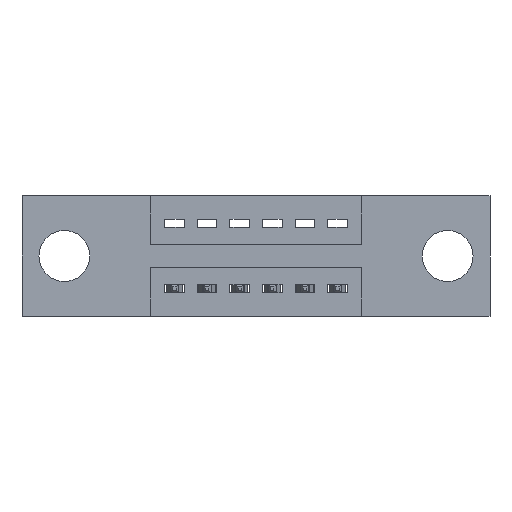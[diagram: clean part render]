
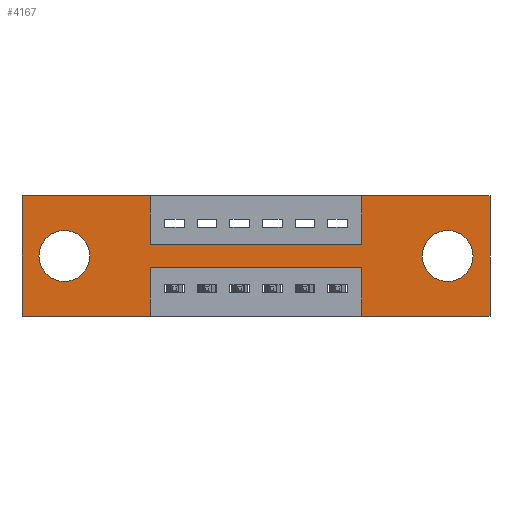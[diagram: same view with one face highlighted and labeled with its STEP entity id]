
A CAD part, front view. The second image highlights one B-rep face of the part: STEP entity #4167.
In plain terms, the highlighted planar face has unit normal (0, -1, 0).
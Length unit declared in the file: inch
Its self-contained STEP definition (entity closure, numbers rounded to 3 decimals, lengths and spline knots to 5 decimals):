
#25 = DIRECTION ( 'NONE',  ( 0., 0., -1. ) ) ;
#95 = EDGE_CURVE ( 'NONE', #3521, #7175, #1944, .T. ) ;
#239 = CIRCLE ( 'NONE', #1973, 0.078 ) ;
#276 = EDGE_CURVE ( 'NONE', #5040, #4251, #2736, .T. ) ;
#314 = LINE ( 'NONE', #8719, #5514 ) ;
#422 = CARTESIAN_POINT ( 'NONE',  ( 0.3925, 0., -0.15 ) ) ;
#449 = EDGE_CURVE ( 'NONE', #4128, #1882, #5234, .T. ) ;
#519 = VECTOR ( 'NONE', #3406, 39.37008 ) ;
#688 = VERTEX_POINT ( 'NONE', #8047 ) ;
#739 = EDGE_CURVE ( 'NONE', #4706, #4128, #9322, .T. ) ;
#760 = CARTESIAN_POINT ( 'NONE',  ( 0.13, 0., -0.107 ) ) ;
#782 = AXIS2_PLACEMENT_3D ( 'NONE', #5456, #6275, #2600 ) ;
#1037 = DIRECTION ( 'NONE',  ( 0., 1., 0. ) ) ;
#1062 = VECTOR ( 'NONE', #7769, 39.37008 ) ;
#1063 = DIRECTION ( 'NONE',  ( 0., 0., 1. ) ) ;
#1074 = CARTESIAN_POINT ( 'NONE',  ( 0.3925, 0., -0.15 ) ) ;
#1185 = VECTOR ( 'NONE', #4696, 39.37008 ) ;
#1388 = EDGE_CURVE ( 'NONE', #6924, #5683, #239, .T. ) ;
#1399 = CARTESIAN_POINT ( 'NONE',  ( 1.435, 0., 0. ) ) ;
#1438 = ORIENTED_EDGE ( 'NONE', *, *, #8268, .F. ) ;
#1604 = DIRECTION ( 'NONE',  ( -1., 0., 0. ) ) ;
#1612 = PLANE ( 'NONE',  #6044 ) ;
#1666 = CIRCLE ( 'NONE', #8547, 0.078 ) ;
#1681 = DIRECTION ( 'NONE',  ( 1., 0., 0. ) ) ;
#1755 = DIRECTION ( 'NONE',  ( 0., 0., -1. ) ) ;
#1757 = ORIENTED_EDGE ( 'NONE', *, *, #1388, .T. ) ;
#1793 = CARTESIAN_POINT ( 'NONE',  ( 1.0425, 0., 0. ) ) ;
#1882 = VERTEX_POINT ( 'NONE', #5999 ) ;
#1934 = VECTOR ( 'NONE', #6250, 39.37008 ) ;
#1942 = CARTESIAN_POINT ( 'NONE',  ( 1.0425, 0., -0.37 ) ) ;
#1944 = LINE ( 'NONE', #9113, #5788 ) ;
#1973 = AXIS2_PLACEMENT_3D ( 'NONE', #6489, #5694, #5533 ) ;
#1988 = ORIENTED_EDGE ( 'NONE', *, *, #3425, .T. ) ;
#2092 = EDGE_LOOP ( 'NONE', ( #8582, #7109 ) ) ;
#2097 = VERTEX_POINT ( 'NONE', #422 ) ;
#2261 = VERTEX_POINT ( 'NONE', #7986 ) ;
#2283 = CARTESIAN_POINT ( 'NONE',  ( 0.13, 0., -0.263 ) ) ;
#2379 = EDGE_CURVE ( 'NONE', #688, #2999, #2798, .T. ) ;
#2382 = CARTESIAN_POINT ( 'NONE',  ( 0., 0., -0.37 ) ) ;
#2531 = ORIENTED_EDGE ( 'NONE', *, *, #739, .F. ) ;
#2545 = DIRECTION ( 'NONE',  ( -1., 0., 0. ) ) ;
#2600 = DIRECTION ( 'NONE',  ( 0., 0., -1. ) ) ;
#2736 = LINE ( 'NONE', #6894, #4638 ) ;
#2756 = LINE ( 'NONE', #4491, #7088 ) ;
#2798 = CIRCLE ( 'NONE', #782, 0.078 ) ;
#2875 = FACE_BOUND ( 'NONE', #3535, .T. ) ;
#2947 = CARTESIAN_POINT ( 'NONE',  ( 0., 0., -0.37 ) ) ;
#2999 = VERTEX_POINT ( 'NONE', #8835 ) ;
#3116 = DIRECTION ( 'NONE',  ( 0., 0., -1. ) ) ;
#3144 = EDGE_CURVE ( 'NONE', #8443, #4706, #314, .T. ) ;
#3175 = DIRECTION ( 'NONE',  ( 0., -1., 0. ) ) ;
#3232 = CARTESIAN_POINT ( 'NONE',  ( 1.0425, 0., -0.15 ) ) ;
#3284 = ORIENTED_EDGE ( 'NONE', *, *, #5875, .F. ) ;
#3406 = DIRECTION ( 'NONE',  ( -1., 0., 0. ) ) ;
#3425 = EDGE_CURVE ( 'NONE', #5683, #6924, #1666, .T. ) ;
#3469 = CARTESIAN_POINT ( 'NONE',  ( 0.3925, 0., -0.37 ) ) ;
#3513 = EDGE_CURVE ( 'NONE', #2999, #688, #6991, .T. ) ;
#3521 = VERTEX_POINT ( 'NONE', #3232 ) ;
#3535 = EDGE_LOOP ( 'NONE', ( #1757, #1988 ) ) ;
#3541 = ORIENTED_EDGE ( 'NONE', *, *, #4475, .F. ) ;
#3552 = LINE ( 'NONE', #7776, #519 ) ;
#3601 = VERTEX_POINT ( 'NONE', #4778 ) ;
#3986 = LINE ( 'NONE', #4208, #4436 ) ;
#4021 = CARTESIAN_POINT ( 'NONE',  ( 0.3925, 0., 0. ) ) ;
#4050 = DIRECTION ( 'NONE',  ( 0., 0., -1. ) ) ;
#4128 = VERTEX_POINT ( 'NONE', #4394 ) ;
#4167 = ADVANCED_FACE ( 'NONE', ( #8006, #2875, #6513 ), #1612, .T. ) ;
#4208 = CARTESIAN_POINT ( 'NONE',  ( 0., 0., 0. ) ) ;
#4251 = VERTEX_POINT ( 'NONE', #9396 ) ;
#4323 = LINE ( 'NONE', #4021, #9220 ) ;
#4363 = ORIENTED_EDGE ( 'NONE', *, *, #276, .F. ) ;
#4394 = CARTESIAN_POINT ( 'NONE',  ( 1.0425, 0., -0.37 ) ) ;
#4436 = VECTOR ( 'NONE', #6277, 39.37008 ) ;
#4439 = ORIENTED_EDGE ( 'NONE', *, *, #3144, .F. ) ;
#4475 = EDGE_CURVE ( 'NONE', #4251, #3601, #3986, .T. ) ;
#4491 = CARTESIAN_POINT ( 'NONE',  ( 0.3925, 0., -0.37 ) ) ;
#4601 = DIRECTION ( 'NONE',  ( 0., 0., 1. ) ) ;
#4638 = VECTOR ( 'NONE', #2545, 39.37008 ) ;
#4686 = EDGE_LOOP ( 'NONE', ( #6322, #7316, #8677, #2531, #4439, #1438, #6793, #8545, #3284, #5772, #3541, #4363 ) ) ;
#4696 = DIRECTION ( 'NONE',  ( 1., 0., 0. ) ) ;
#4706 = VERTEX_POINT ( 'NONE', #7402 ) ;
#4778 = CARTESIAN_POINT ( 'NONE',  ( 0., 0., 0. ) ) ;
#4788 = LINE ( 'NONE', #1074, #1185 ) ;
#4893 = VECTOR ( 'NONE', #1681, 39.37008 ) ;
#5040 = VERTEX_POINT ( 'NONE', #3469 ) ;
#5069 = AXIS2_PLACEMENT_3D ( 'NONE', #5360, #1037, #1755 ) ;
#5234 = LINE ( 'NONE', #1942, #1934 ) ;
#5360 = CARTESIAN_POINT ( 'NONE',  ( 1.305, 0., -0.185 ) ) ;
#5456 = CARTESIAN_POINT ( 'NONE',  ( 1.305, 0., -0.185 ) ) ;
#5492 = CARTESIAN_POINT ( 'NONE',  ( 0., 0., 0. ) ) ;
#5514 = VECTOR ( 'NONE', #25, 39.37008 ) ;
#5533 = DIRECTION ( 'NONE',  ( 0., 0., 1. ) ) ;
#5683 = VERTEX_POINT ( 'NONE', #2283 ) ;
#5694 = DIRECTION ( 'NONE',  ( 0., 1., 0. ) ) ;
#5772 = ORIENTED_EDGE ( 'NONE', *, *, #8872, .F. ) ;
#5788 = VECTOR ( 'NONE', #4601, 39.37008 ) ;
#5875 = EDGE_CURVE ( 'NONE', #9173, #2097, #4323, .T. ) ;
#5999 = CARTESIAN_POINT ( 'NONE',  ( 1.0425, 0., -0.22 ) ) ;
#6044 = AXIS2_PLACEMENT_3D ( 'NONE', #2382, #3175, #4050 ) ;
#6250 = DIRECTION ( 'NONE',  ( 0., 0., 1. ) ) ;
#6260 = LINE ( 'NONE', #8830, #4893 ) ;
#6275 = DIRECTION ( 'NONE',  ( 0., 1., 0. ) ) ;
#6277 = DIRECTION ( 'NONE',  ( 0., 0., 1. ) ) ;
#6322 = ORIENTED_EDGE ( 'NONE', *, *, #7971, .F. ) ;
#6489 = CARTESIAN_POINT ( 'NONE',  ( 0.13, 0., -0.185 ) ) ;
#6513 = FACE_OUTER_BOUND ( 'NONE', #4686, .T. ) ;
#6793 = ORIENTED_EDGE ( 'NONE', *, *, #95, .F. ) ;
#6890 = DIRECTION ( 'NONE',  ( 0., 1., 0. ) ) ;
#6894 = CARTESIAN_POINT ( 'NONE',  ( 0., 0., -0.37 ) ) ;
#6924 = VERTEX_POINT ( 'NONE', #760 ) ;
#6991 = CIRCLE ( 'NONE', #5069, 0.078 ) ;
#7088 = VECTOR ( 'NONE', #3116, 39.37008 ) ;
#7109 = ORIENTED_EDGE ( 'NONE', *, *, #2379, .T. ) ;
#7168 = VECTOR ( 'NONE', #1604, 39.37008 ) ;
#7175 = VERTEX_POINT ( 'NONE', #1793 ) ;
#7186 = LINE ( 'NONE', #5492, #1062 ) ;
#7316 = ORIENTED_EDGE ( 'NONE', *, *, #7683, .F. ) ;
#7402 = CARTESIAN_POINT ( 'NONE',  ( 1.435, 0., -0.37 ) ) ;
#7669 = EDGE_CURVE ( 'NONE', #2097, #3521, #4788, .T. ) ;
#7683 = EDGE_CURVE ( 'NONE', #1882, #2261, #3552, .T. ) ;
#7769 = DIRECTION ( 'NONE',  ( 1., 0., 0. ) ) ;
#7776 = CARTESIAN_POINT ( 'NONE',  ( 0.3925, 0., -0.22 ) ) ;
#7971 = EDGE_CURVE ( 'NONE', #2261, #5040, #2756, .T. ) ;
#7986 = CARTESIAN_POINT ( 'NONE',  ( 0.3925, 0., -0.22 ) ) ;
#8006 = FACE_BOUND ( 'NONE', #2092, .T. ) ;
#8047 = CARTESIAN_POINT ( 'NONE',  ( 1.305, 0., -0.263 ) ) ;
#8268 = EDGE_CURVE ( 'NONE', #7175, #8443, #7186, .T. ) ;
#8443 = VERTEX_POINT ( 'NONE', #1399 ) ;
#8533 = DIRECTION ( 'NONE',  ( 0., 0., -1. ) ) ;
#8545 = ORIENTED_EDGE ( 'NONE', *, *, #7669, .F. ) ;
#8547 = AXIS2_PLACEMENT_3D ( 'NONE', #9094, #6890, #1063 ) ;
#8582 = ORIENTED_EDGE ( 'NONE', *, *, #3513, .T. ) ;
#8677 = ORIENTED_EDGE ( 'NONE', *, *, #449, .F. ) ;
#8719 = CARTESIAN_POINT ( 'NONE',  ( 1.435, 0., 0. ) ) ;
#8830 = CARTESIAN_POINT ( 'NONE',  ( 0., 0., 0. ) ) ;
#8835 = CARTESIAN_POINT ( 'NONE',  ( 1.305, 0., -0.107 ) ) ;
#8872 = EDGE_CURVE ( 'NONE', #3601, #9173, #6260, .T. ) ;
#9094 = CARTESIAN_POINT ( 'NONE',  ( 0.13, 0., -0.185 ) ) ;
#9113 = CARTESIAN_POINT ( 'NONE',  ( 1.0425, 0., 0. ) ) ;
#9173 = VERTEX_POINT ( 'NONE', #9240 ) ;
#9220 = VECTOR ( 'NONE', #8533, 39.37008 ) ;
#9240 = CARTESIAN_POINT ( 'NONE',  ( 0.3925, 0., 0. ) ) ;
#9322 = LINE ( 'NONE', #2947, #7168 ) ;
#9396 = CARTESIAN_POINT ( 'NONE',  ( 0., 0., -0.37 ) ) ;
